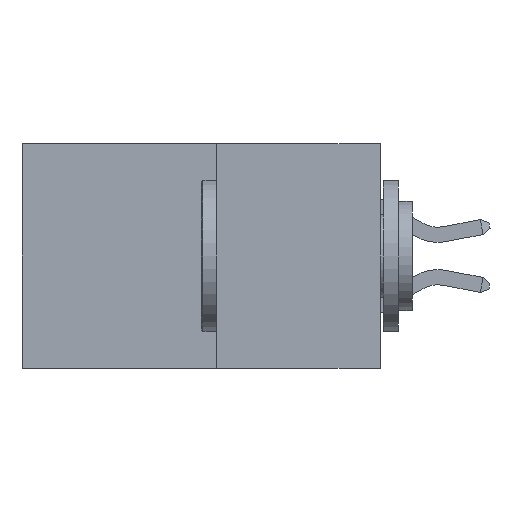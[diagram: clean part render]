
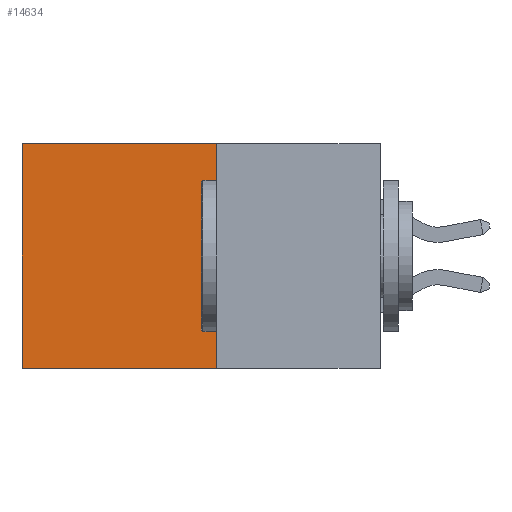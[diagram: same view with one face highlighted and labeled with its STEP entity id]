
A CAD part, left-side view. The second image highlights one B-rep face of the part: STEP entity #14634.
In plain terms, the highlighted planar face has unit normal (-1, 0, 0).
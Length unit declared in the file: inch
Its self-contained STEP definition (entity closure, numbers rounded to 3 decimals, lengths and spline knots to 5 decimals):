
#1018 = EDGE_CURVE ( 'NONE', #1836, #7619, #4216, .T. ) ;
#1633 = VECTOR ( 'NONE', #18056, 39.37008 ) ;
#1836 = VERTEX_POINT ( 'NONE', #18796 ) ;
#1885 = EDGE_CURVE ( 'NONE', #8247, #7619, #13767, .T. ) ;
#2196 = CARTESIAN_POINT ( 'NONE',  ( 0.277, 0.27, -0.37 ) ) ;
#3751 = DIRECTION ( 'NONE',  ( 0., 0., -1. ) ) ;
#4216 = LINE ( 'NONE', #6764, #11831 ) ;
#4347 = CARTESIAN_POINT ( 'NONE',  ( 0.277, 0.27, -0.37 ) ) ;
#5088 = ORIENTED_EDGE ( 'NONE', *, *, #15456, .T. ) ;
#5831 = CARTESIAN_POINT ( 'NONE',  ( 0.277, 0.27, -0.37 ) ) ;
#6020 = CARTESIAN_POINT ( 'NONE',  ( 0.277, 0.27, 0. ) ) ;
#6165 = ORIENTED_EDGE ( 'NONE', *, *, #10156, .F. ) ;
#6482 = ORIENTED_EDGE ( 'NONE', *, *, #1885, .F. ) ;
#6587 = LINE ( 'NONE', #19306, #14581 ) ;
#6736 = DIRECTION ( 'NONE',  ( 0., 0., -1. ) ) ;
#6764 = CARTESIAN_POINT ( 'NONE',  ( 0.277, 0.59, -0.37 ) ) ;
#7619 = VERTEX_POINT ( 'NONE', #14207 ) ;
#8247 = VERTEX_POINT ( 'NONE', #5831 ) ;
#8416 = ORIENTED_EDGE ( 'NONE', *, *, #1018, .T. ) ;
#9279 = FACE_OUTER_BOUND ( 'NONE', #19145, .T. ) ;
#10156 = EDGE_CURVE ( 'NONE', #13491, #8247, #19048, .T. ) ;
#11628 = AXIS2_PLACEMENT_3D ( 'NONE', #2196, #12856, #3751 ) ;
#11831 = VECTOR ( 'NONE', #6736, 39.37008 ) ;
#11923 = DIRECTION ( 'NONE',  ( 0., 1., 0. ) ) ;
#12856 = DIRECTION ( 'NONE',  ( 1., 0., 0. ) ) ;
#13491 = VERTEX_POINT ( 'NONE', #6020 ) ;
#13767 = LINE ( 'NONE', #17672, #1633 ) ;
#14207 = CARTESIAN_POINT ( 'NONE',  ( 0.277, 0.59, -0.37 ) ) ;
#14581 = VECTOR ( 'NONE', #11923, 39.37008 ) ;
#14634 = ADVANCED_FACE ( 'NONE', ( #9279 ), #17260, .F. ) ;
#14906 = DIRECTION ( 'NONE',  ( 0., 0., -1. ) ) ;
#15456 = EDGE_CURVE ( 'NONE', #13491, #1836, #6587, .T. ) ;
#15574 = VECTOR ( 'NONE', #14906, 39.37008 ) ;
#17260 = PLANE ( 'NONE',  #11628 ) ;
#17672 = CARTESIAN_POINT ( 'NONE',  ( 0.277, 0.27, -0.37 ) ) ;
#18056 = DIRECTION ( 'NONE',  ( 0., 1., 0. ) ) ;
#18796 = CARTESIAN_POINT ( 'NONE',  ( 0.277, 0.59, 0. ) ) ;
#19048 = LINE ( 'NONE', #4347, #15574 ) ;
#19145 = EDGE_LOOP ( 'NONE', ( #8416, #6482, #6165, #5088 ) ) ;
#19306 = CARTESIAN_POINT ( 'NONE',  ( 0.277, 0.27, 0. ) ) ;
